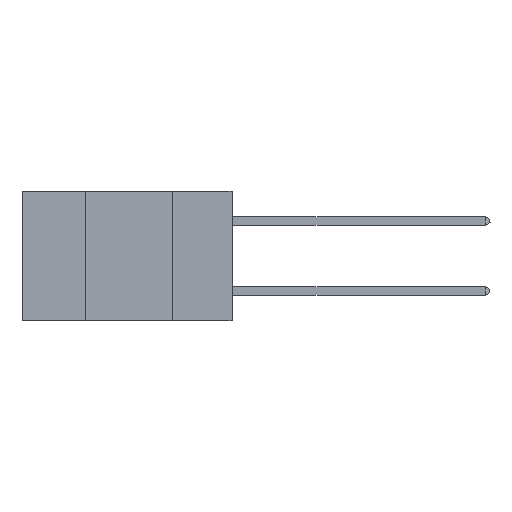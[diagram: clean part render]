
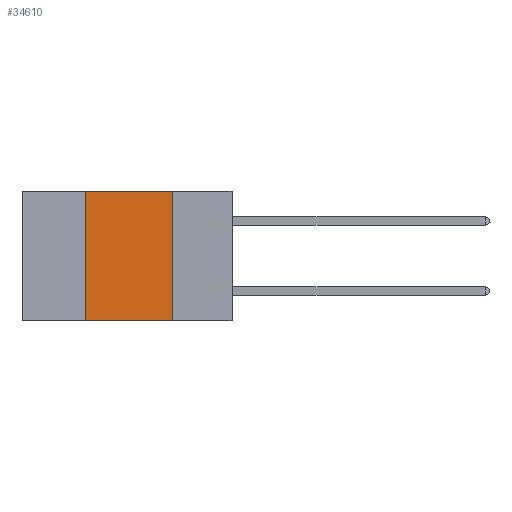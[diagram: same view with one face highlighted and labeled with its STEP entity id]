
A CAD part, left-side view. The second image highlights one B-rep face of the part: STEP entity #34610.
In plain terms, the highlighted planar face has unit normal (-1, 0, 0).
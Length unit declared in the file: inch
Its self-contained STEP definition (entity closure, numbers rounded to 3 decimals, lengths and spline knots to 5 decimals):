
#166 = CARTESIAN_POINT ( 'NONE',  ( 0., 0.6, 0. ) ) ;
#2145 = VECTOR ( 'NONE', #8017, 39.37008 ) ;
#3810 = CARTESIAN_POINT ( 'NONE',  ( 0., 0.42, -0.37 ) ) ;
#3868 = EDGE_CURVE ( 'NONE', #6432, #31403, #34749, .T. ) ;
#3878 = CARTESIAN_POINT ( 'NONE',  ( 0., 0.42, 0. ) ) ;
#3917 = FACE_OUTER_BOUND ( 'NONE', #41002, .T. ) ;
#5226 = CARTESIAN_POINT ( 'NONE',  ( 0., 0.17, 0. ) ) ;
#5641 = AXIS2_PLACEMENT_3D ( 'NONE', #166, #23352, #36645 ) ;
#6432 = VERTEX_POINT ( 'NONE', #20624 ) ;
#8017 = DIRECTION ( 'NONE',  ( 0., -1., 0. ) ) ;
#8404 = VERTEX_POINT ( 'NONE', #14738 ) ;
#9940 = PLANE ( 'NONE',  #5641 ) ;
#10873 = LINE ( 'NONE', #5226, #11902 ) ;
#11902 = VECTOR ( 'NONE', #35200, 39.37008 ) ;
#12047 = VERTEX_POINT ( 'NONE', #3810 ) ;
#14299 = DIRECTION ( 'NONE',  ( 0., -1., 0. ) ) ;
#14738 = CARTESIAN_POINT ( 'NONE',  ( 0., 0.17, -0.37 ) ) ;
#15230 = ORIENTED_EDGE ( 'NONE', *, *, #28108, .T. ) ;
#15972 = ORIENTED_EDGE ( 'NONE', *, *, #31386, .F. ) ;
#18702 = VECTOR ( 'NONE', #14299, 39.37008 ) ;
#18739 = LINE ( 'NONE', #41073, #2145 ) ;
#20624 = CARTESIAN_POINT ( 'NONE',  ( 0., 0.42, 0. ) ) ;
#23352 = DIRECTION ( 'NONE',  ( 1., 0., 0. ) ) ;
#23378 = ORIENTED_EDGE ( 'NONE', *, *, #3868, .F. ) ;
#24700 = EDGE_CURVE ( 'NONE', #12047, #6432, #29612, .T. ) ;
#26547 = VECTOR ( 'NONE', #36765, 39.37008 ) ;
#27366 = CARTESIAN_POINT ( 'NONE',  ( 0., 0.6, 0. ) ) ;
#28108 = EDGE_CURVE ( 'NONE', #12047, #8404, #18739, .T. ) ;
#29612 = LINE ( 'NONE', #3878, #26547 ) ;
#31386 = EDGE_CURVE ( 'NONE', #31403, #8404, #10873, .T. ) ;
#31403 = VERTEX_POINT ( 'NONE', #31867 ) ;
#31867 = CARTESIAN_POINT ( 'NONE',  ( 0., 0.17, 0. ) ) ;
#34610 = ADVANCED_FACE ( 'NONE', ( #3917 ), #9940, .F. ) ;
#34749 = LINE ( 'NONE', #27366, #18702 ) ;
#35200 = DIRECTION ( 'NONE',  ( 0., 0., -1. ) ) ;
#36645 = DIRECTION ( 'NONE',  ( 0., 0., -1. ) ) ;
#36765 = DIRECTION ( 'NONE',  ( 0., 0., 1. ) ) ;
#36996 = ORIENTED_EDGE ( 'NONE', *, *, #24700, .F. ) ;
#41002 = EDGE_LOOP ( 'NONE', ( #15972, #23378, #36996, #15230 ) ) ;
#41073 = CARTESIAN_POINT ( 'NONE',  ( 0., 0.6, -0.37 ) ) ;
